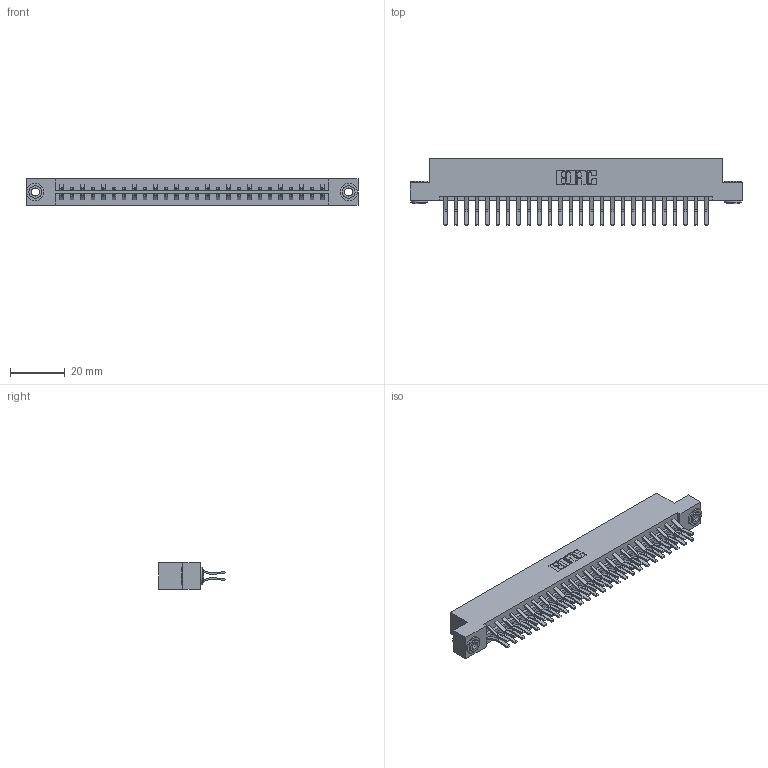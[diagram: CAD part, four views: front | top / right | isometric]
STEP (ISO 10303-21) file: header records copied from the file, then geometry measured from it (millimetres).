
FILE_DESCRIPTION (( 'STEP AP203' ), '1' );
FILE_NAME ('379-052-560-203.STEP', '2020-02-26T18:16:28', ( '' ), ( '' ), 'SwSTEP 2.0', 'SolidWorks 2016', '' );
FILE_SCHEMA (( 'CONFIG_CONTROL_DESIGN' ));
Length unit declared in the file: inch
Products named in the file (4): 345-250-002_345-250-002-102; 345-292-001_560 Tail; 379-052-560-203; 379 Part_Flush - .156 Dia - TH
Assembly tree (55 placements, depth 2):
  379-052-560-203
    379 Part_Flush - .156 Dia - TH
    345-292-001_560 Tail  x52
    345-250-002_345-250-002-102  x2
Bounding box: 121.28 x 24.45 x 9.53 mm (x, y, z)
Volume: 13082.4 mm3; surface area: 15760.8 mm2
Topology: 55 solids, 55 shells, 2960 faces, 8759 edges, 5766 vertices
Faces by surface type: plane 1952, cylinder 1000, cone 8
Entity records: 19534 total; most frequent: CARTESIAN_POINT 3233, ORIENTED_EDGE 3162, DIRECTION 2827, EDGE_CURVE 1581, VECTOR 1425, LINE 1425, VERTEX_POINT 1050, AXIS2_PLACEMENT_3D 701
